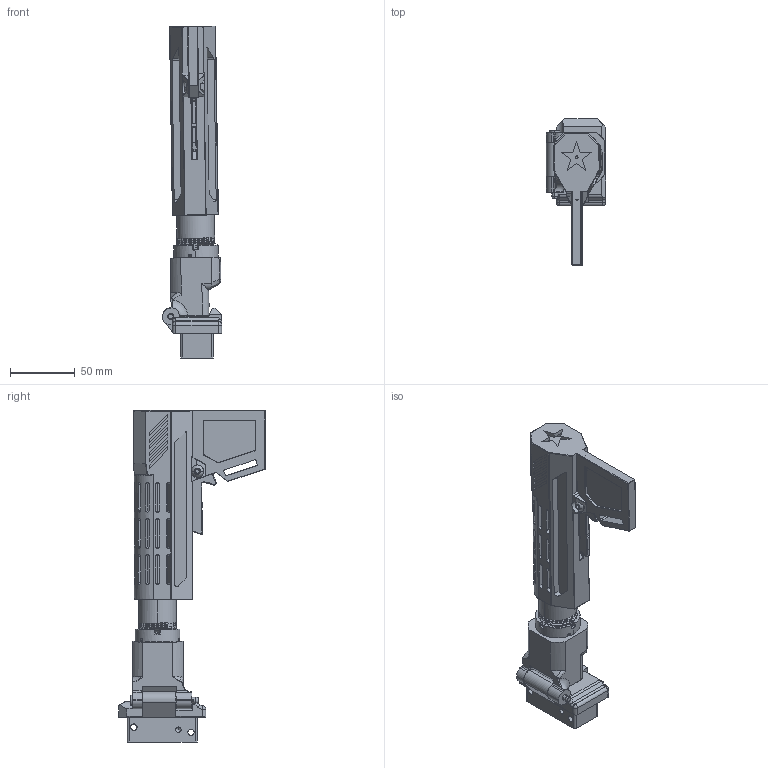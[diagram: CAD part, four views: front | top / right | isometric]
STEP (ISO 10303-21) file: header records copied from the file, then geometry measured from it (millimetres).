
FILE_DESCRIPTION (( 'STEP AP214' ), '1' );
FILE_NAME ('PPDW9 V4 Folding Buffer.STEP', '2020-12-31T21:10:15', ( '' ), ( '' ), 'SwSTEP 2.0', 'SolidWorks 2020', '' );
FILE_SCHEMA (( 'AUTOMOTIVE_DESIGN' ));
Length unit declared in the file: inch
Products named in the file (13): Buffer Tube Nut; Buffer Tube Mil Spec; PPDW9 V2 Buffer tube adapter; PPDW9 V4 Folding Buffer; PPDW9 V4 Modcat folding buffer tube endcap; KEKwave for MilSpec tube; 90156A212_QUICK-RELEASE CLEVIS PIN WITH HEAD_90156A212; KEKwave lock tab milspec buffer tube; Folding brace Button; M5 nut 98676A300_98676A300; UMP SB Tactical spring_9662K22; M5 x 12mm BHSH 91239A228_BLACK_91239A228; Spring Kek mil spec lever lock 9435K180_9435K18
Assembly tree (12 placements, depth 2):
  PPDW9 V4 Folding Buffer
    PPDW9 V4 Modcat folding buffer tube endcap
    Folding brace Button
    PPDW9 V2 Buffer tube adapter
    Buffer Tube Mil Spec
    Buffer Tube Nut
    KEKwave for MilSpec tube
    KEKwave lock tab milspec buffer tube
    90156A212_QUICK-RELEASE CLEVIS PIN WITH HEAD_90156A212
    Spring Kek mil spec lever lock 9435K180_9435K18
    M5 x 12mm BHSH 91239A228_BLACK_91239A228
    M5 nut 98676A300_98676A300
    UMP SB Tactical spring_9662K22
Bounding box: 45.97 x 113.72 x 257.24 mm (x, y, z)
Volume: 224824.2 mm3; surface area: 126167.2 mm2
Topology: 13 solids, 22 shells, 1669 faces, 4473 edges, 2811 vertices
Faces by surface type: cylinder 609, plane 553, bspline 363, torus 54, cone 50, sphere 40
Entity records: 118494 total; most frequent: CARTESIAN_POINT 80072, ORIENTED_EDGE 8818, DIRECTION 6163, EDGE_CURVE 4409, VERTEX_POINT 2802, AXIS2_PLACEMENT_3D 2087, LINE 1989, VECTOR 1989
